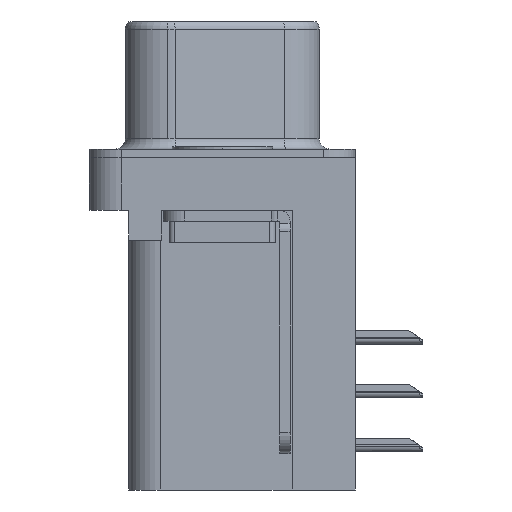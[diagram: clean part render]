
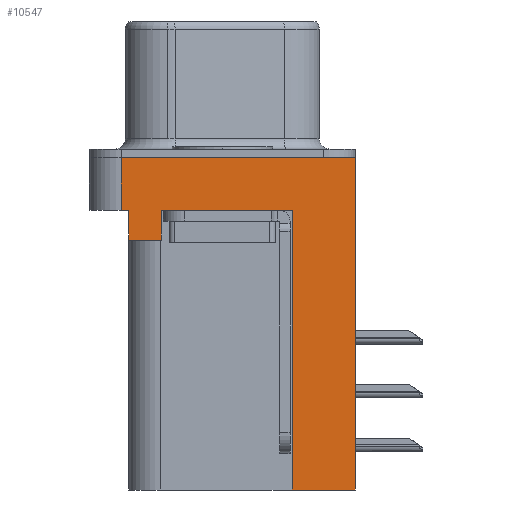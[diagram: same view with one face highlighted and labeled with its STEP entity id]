
A CAD part, left-side view. The second image highlights one B-rep face of the part: STEP entity #10547.
In plain terms, the highlighted planar face has unit normal (-1, 0, 0).
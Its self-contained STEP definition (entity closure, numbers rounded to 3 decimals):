
#77 = VECTOR ( 'NONE', #21054, 1000. ) ;
#152 = VERTEX_POINT ( 'NONE', #22179 ) ;
#1197 = LINE ( 'NONE', #12438, #6741 ) ;
#1530 = CARTESIAN_POINT ( 'NONE',  ( -3., 2.895, -2.5 ) ) ;
#1663 = LINE ( 'NONE', #26509, #7867 ) ;
#2010 = EDGE_CURVE ( 'NONE', #16038, #15067, #1197, .T. ) ;
#2314 = ORIENTED_EDGE ( 'NONE', *, *, #15892, .F. ) ;
#2321 = VERTEX_POINT ( 'NONE', #24918 ) ;
#3160 = DIRECTION ( 'NONE',  ( 0., 0., 1. ) ) ;
#3254 = EDGE_CURVE ( 'NONE', #5347, #22795, #20484, .T. ) ;
#4304 = DIRECTION ( 'NONE',  ( 0., 0., 1. ) ) ;
#4309 = DIRECTION ( 'NONE',  ( 0., 1., 0. ) ) ;
#4465 = CARTESIAN_POINT ( 'NONE',  ( -3., -6.275, -2.5 ) ) ;
#4866 = ORIENTED_EDGE ( 'NONE', *, *, #12226, .T. ) ;
#4945 = CARTESIAN_POINT ( 'NONE',  ( -3., -3.295, -2.5 ) ) ;
#4972 = ORIENTED_EDGE ( 'NONE', *, *, #24554, .T. ) ;
#5347 = VERTEX_POINT ( 'NONE', #20091 ) ;
#5360 = CARTESIAN_POINT ( 'NONE',  ( -3., -6.275, 0. ) ) ;
#5372 = ORIENTED_EDGE ( 'NONE', *, *, #12815, .F. ) ;
#5416 = VECTOR ( 'NONE', #25553, 1000. ) ;
#6436 = CARTESIAN_POINT ( 'NONE',  ( -3., -3.295, -15.7 ) ) ;
#6600 = LINE ( 'NONE', #14405, #17113 ) ;
#6707 = DIRECTION ( 'NONE',  ( 0., 0., 1. ) ) ;
#6741 = VECTOR ( 'NONE', #13469, 1000. ) ;
#6773 = FACE_OUTER_BOUND ( 'NONE', #25598, .T. ) ;
#7569 = CARTESIAN_POINT ( 'NONE',  ( -3., 4.775, -2.5 ) ) ;
#7867 = VECTOR ( 'NONE', #11759, 1000. ) ;
#8802 = CARTESIAN_POINT ( 'NONE',  ( -3., 4.775, -2.5 ) ) ;
#9989 = CARTESIAN_POINT ( 'NONE',  ( -3., -3.295, -15.7 ) ) ;
#10380 = VECTOR ( 'NONE', #6707, 1000. ) ;
#10547 = ADVANCED_FACE ( 'NONE', ( #6773 ), #11510, .T. ) ;
#11280 = ORIENTED_EDGE ( 'NONE', *, *, #25726, .F. ) ;
#11510 = PLANE ( 'NONE',  #12904 ) ;
#11759 = DIRECTION ( 'NONE',  ( 0., 1., 0. ) ) ;
#12226 = EDGE_CURVE ( 'NONE', #15067, #18316, #22163, .T. ) ;
#12410 = ORIENTED_EDGE ( 'NONE', *, *, #2010, .T. ) ;
#12438 = CARTESIAN_POINT ( 'NONE',  ( -3., 2.895, -3.9 ) ) ;
#12541 = CARTESIAN_POINT ( 'NONE',  ( -3., 4.425, -3.9 ) ) ;
#12815 = EDGE_CURVE ( 'NONE', #152, #2321, #18854, .T. ) ;
#12904 = AXIS2_PLACEMENT_3D ( 'NONE', #13632, #15730, #3160 ) ;
#13044 = CARTESIAN_POINT ( 'NONE',  ( -3., -6.275, 0. ) ) ;
#13469 = DIRECTION ( 'NONE',  ( 0., 0., 1. ) ) ;
#13632 = CARTESIAN_POINT ( 'NONE',  ( -3., -6.275, -2.5 ) ) ;
#13856 = EDGE_CURVE ( 'NONE', #16038, #152, #1663, .T. ) ;
#14405 = CARTESIAN_POINT ( 'NONE',  ( -3., -6.275, -2.5 ) ) ;
#14778 = CARTESIAN_POINT ( 'NONE',  ( -3., -3.295, -15.7 ) ) ;
#14911 = VECTOR ( 'NONE', #15176, 1000. ) ;
#15067 = VERTEX_POINT ( 'NONE', #1530 ) ;
#15176 = DIRECTION ( 'NONE',  ( 0., -1., 0. ) ) ;
#15730 = DIRECTION ( 'NONE',  ( -1., 0., 0. ) ) ;
#15881 = LINE ( 'NONE', #4465, #26454 ) ;
#15892 = EDGE_CURVE ( 'NONE', #22330, #24340, #16325, .T. ) ;
#15968 = LINE ( 'NONE', #8802, #10380 ) ;
#16038 = VERTEX_POINT ( 'NONE', #23657 ) ;
#16290 = VERTEX_POINT ( 'NONE', #7569 ) ;
#16325 = LINE ( 'NONE', #14778, #21245 ) ;
#17113 = VECTOR ( 'NONE', #18603, 1000. ) ;
#18199 = VECTOR ( 'NONE', #4304, 1000. ) ;
#18316 = VERTEX_POINT ( 'NONE', #4945 ) ;
#18603 = DIRECTION ( 'NONE',  ( 0., -1., 0. ) ) ;
#18854 = LINE ( 'NONE', #12541, #18199 ) ;
#20091 = CARTESIAN_POINT ( 'NONE',  ( -3., 4.775, 0. ) ) ;
#20171 = ORIENTED_EDGE ( 'NONE', *, *, #26655, .T. ) ;
#20484 = LINE ( 'NONE', #13044, #14911 ) ;
#21054 = DIRECTION ( 'NONE',  ( 0., 0., 1. ) ) ;
#21245 = VECTOR ( 'NONE', #4309, 1000. ) ;
#21539 = ORIENTED_EDGE ( 'NONE', *, *, #23152, .F. ) ;
#22163 = LINE ( 'NONE', #23398, #5416 ) ;
#22179 = CARTESIAN_POINT ( 'NONE',  ( -3., 4.425, -3.9 ) ) ;
#22330 = VERTEX_POINT ( 'NONE', #24775 ) ;
#22388 = LINE ( 'NONE', #6436, #77 ) ;
#22795 = VERTEX_POINT ( 'NONE', #5360 ) ;
#22901 = ORIENTED_EDGE ( 'NONE', *, *, #3254, .F. ) ;
#23152 = EDGE_CURVE ( 'NONE', #16290, #5347, #15968, .T. ) ;
#23370 = DIRECTION ( 'NONE',  ( 0., 0., 1. ) ) ;
#23398 = CARTESIAN_POINT ( 'NONE',  ( -3., -6.275, -2.5 ) ) ;
#23657 = CARTESIAN_POINT ( 'NONE',  ( -3., 2.895, -3.9 ) ) ;
#24340 = VERTEX_POINT ( 'NONE', #9989 ) ;
#24554 = EDGE_CURVE ( 'NONE', #22330, #22795, #15881, .T. ) ;
#24708 = ORIENTED_EDGE ( 'NONE', *, *, #13856, .F. ) ;
#24775 = CARTESIAN_POINT ( 'NONE',  ( -3., -6.275, -15.7 ) ) ;
#24918 = CARTESIAN_POINT ( 'NONE',  ( -3., 4.425, -2.5 ) ) ;
#25553 = DIRECTION ( 'NONE',  ( 0., -1., 0. ) ) ;
#25598 = EDGE_LOOP ( 'NONE', ( #22901, #21539, #20171, #5372, #24708, #12410, #4866, #11280, #2314, #4972 ) ) ;
#25726 = EDGE_CURVE ( 'NONE', #24340, #18316, #22388, .T. ) ;
#26454 = VECTOR ( 'NONE', #23370, 1000. ) ;
#26509 = CARTESIAN_POINT ( 'NONE',  ( -3., 4.425, -3.9 ) ) ;
#26655 = EDGE_CURVE ( 'NONE', #16290, #2321, #6600, .T. ) ;
